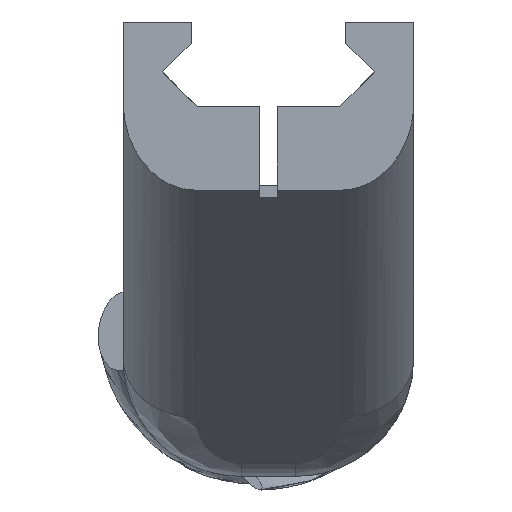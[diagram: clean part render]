
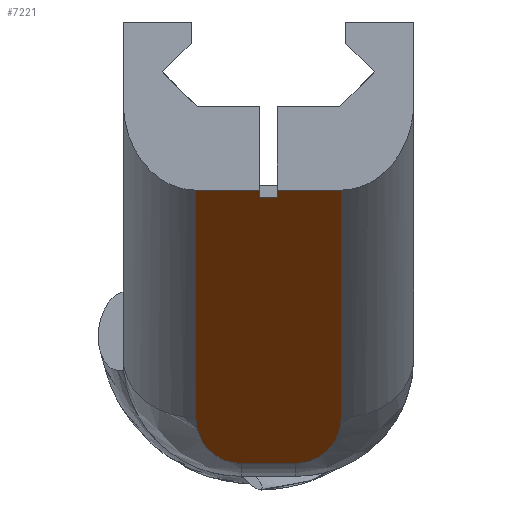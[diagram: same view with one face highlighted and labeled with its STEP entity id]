
A CAD part, front view. The second image highlights one B-rep face of the part: STEP entity #7221.
In plain terms, the highlighted planar face has unit normal (0, -0.574, -0.819).
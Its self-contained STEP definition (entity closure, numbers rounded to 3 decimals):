
#200 = EDGE_CURVE ( 'NONE', #5233, #2700, #1106, .T. ) ;
#331 = CARTESIAN_POINT ( 'NONE',  ( 8., 39.963, -21.482 ) ) ;
#423 = CARTESIAN_POINT ( 'NONE',  ( -1., 1.18, 5.674 ) ) ;
#667 = VERTEX_POINT ( 'NONE', #8123 ) ;
#801 = CARTESIAN_POINT ( 'NONE',  ( 16., 1.18, 5.674 ) ) ;
#875 = CARTESIAN_POINT ( 'NONE',  ( 16., 0., 6.5 ) ) ;
#878 = VECTOR ( 'NONE', #1994, 1000. ) ;
#936 = LINE ( 'NONE', #875, #3476 ) ;
#1106 =( BOUNDED_CURVE ( )  B_SPLINE_CURVE ( 3, ( #1747, #4304, #6349, #9947 ),
 .UNSPECIFIED., .F., .T. ) 
 B_SPLINE_CURVE_WITH_KNOTS ( ( 4, 4 ),
 ( 1.571, 3.142 ),
 .UNSPECIFIED. ) 
 CURVE ( )  GEOMETRIC_REPRESENTATION_ITEM ( )  RATIONAL_B_SPLINE_CURVE ( ( 1., 0.805, 0.805, 1. ) ) 
 REPRESENTATION_ITEM ( '' )  );
#1144 = CARTESIAN_POINT ( 'NONE',  ( 5.929, 42.92, -23.553 ) ) ;
#1277 = AXIS2_PLACEMENT_3D ( 'NONE', #10668, #2596, #5287 ) ;
#1302 = CARTESIAN_POINT ( 'NONE',  ( 3., 42.92, -23.553 ) ) ;
#1432 = VERTEX_POINT ( 'NONE', #423 ) ;
#1663 = ORIENTED_EDGE ( 'NONE', *, *, #2831, .T. ) ;
#1701 = DIRECTION ( 'NONE',  ( -1., 0., 0. ) ) ;
#1747 = CARTESIAN_POINT ( 'NONE',  ( -8., 35.78, -18.553 ) ) ;
#1974 = DIRECTION ( 'NONE',  ( 0., -0.819, 0.574 ) ) ;
#1994 = DIRECTION ( 'NONE',  ( 1., 0., 0. ) ) ;
#2178 =( BOUNDED_CURVE ( )  B_SPLINE_CURVE ( 3, ( #6588, #1144, #331, #3803 ),
 .UNSPECIFIED., .F., .T. ) 
 B_SPLINE_CURVE_WITH_KNOTS ( ( 4, 4 ),
 ( 0., 1.571 ),
 .UNSPECIFIED. ) 
 CURVE ( )  GEOMETRIC_REPRESENTATION_ITEM ( )  RATIONAL_B_SPLINE_CURVE ( ( 1., 0.805, 0.805, 1. ) ) 
 REPRESENTATION_ITEM ( '' )  );
#2285 = CARTESIAN_POINT ( 'NONE',  ( 1., 0., 6.5 ) ) ;
#2437 = CARTESIAN_POINT ( 'NONE',  ( 16., 0., 6.5 ) ) ;
#2596 = DIRECTION ( 'NONE',  ( 0., 0.574, 0.819 ) ) ;
#2638 = EDGE_CURVE ( 'NONE', #667, #7764, #2783, .T. ) ;
#2700 = VERTEX_POINT ( 'NONE', #7152 ) ;
#2783 = LINE ( 'NONE', #5602, #3852 ) ;
#2831 = EDGE_CURVE ( 'NONE', #9083, #7705, #2854, .T. ) ;
#2854 = LINE ( 'NONE', #7446, #9708 ) ;
#3458 = VERTEX_POINT ( 'NONE', #11297 ) ;
#3476 = VECTOR ( 'NONE', #1701, 1000. ) ;
#3803 = CARTESIAN_POINT ( 'NONE',  ( 8., 35.78, -18.553 ) ) ;
#3852 = VECTOR ( 'NONE', #1974, 1000. ) ;
#4027 = VECTOR ( 'NONE', #5183, 1000. ) ;
#4177 = DIRECTION ( 'NONE',  ( 1., 0., 0. ) ) ;
#4202 = EDGE_CURVE ( 'NONE', #2700, #7666, #10027, .T. ) ;
#4281 = EDGE_CURVE ( 'NONE', #7764, #9083, #936, .T. ) ;
#4304 = CARTESIAN_POINT ( 'NONE',  ( -8., 39.963, -21.482 ) ) ;
#4727 = DIRECTION ( 'NONE',  ( 0., 0.819, -0.574 ) ) ;
#4997 = EDGE_CURVE ( 'NONE', #1432, #7705, #11282, .T. ) ;
#5050 = ORIENTED_EDGE ( 'NONE', *, *, #2638, .T. ) ;
#5065 = EDGE_CURVE ( 'NONE', #5822, #3458, #9645, .T. ) ;
#5183 = DIRECTION ( 'NONE',  ( -1., 0., 0. ) ) ;
#5233 = VERTEX_POINT ( 'NONE', #8159 ) ;
#5287 = DIRECTION ( 'NONE',  ( 0., -0.819, 0.574 ) ) ;
#5555 = VECTOR ( 'NONE', #7245, 1000. ) ;
#5602 = CARTESIAN_POINT ( 'NONE',  ( 8., 50., -28.51 ) ) ;
#5822 = VERTEX_POINT ( 'NONE', #10461 ) ;
#6167 = FACE_OUTER_BOUND ( 'NONE', #9370, .T. ) ;
#6207 = CARTESIAN_POINT ( 'NONE',  ( 8., 0., 6.5 ) ) ;
#6349 = CARTESIAN_POINT ( 'NONE',  ( -5.929, 42.92, -23.553 ) ) ;
#6436 = LINE ( 'NONE', #8928, #6712 ) ;
#6588 = CARTESIAN_POINT ( 'NONE',  ( 3., 42.92, -23.553 ) ) ;
#6712 = VECTOR ( 'NONE', #11313, 1000. ) ;
#6910 = ORIENTED_EDGE ( 'NONE', *, *, #5065, .T. ) ;
#6945 = ORIENTED_EDGE ( 'NONE', *, *, #4281, .T. ) ;
#7152 = CARTESIAN_POINT ( 'NONE',  ( -3., 42.92, -23.553 ) ) ;
#7221 = ADVANCED_FACE ( 'NONE', ( #6167 ), #10605, .F. ) ;
#7245 = DIRECTION ( 'NONE',  ( 0., 0.819, -0.574 ) ) ;
#7446 = CARTESIAN_POINT ( 'NONE',  ( 1., 50., -28.51 ) ) ;
#7520 = EDGE_CURVE ( 'NONE', #3458, #5233, #11586, .T. ) ;
#7627 = VECTOR ( 'NONE', #4177, 1000. ) ;
#7666 = VERTEX_POINT ( 'NONE', #9731 ) ;
#7705 = VERTEX_POINT ( 'NONE', #10064 ) ;
#7764 = VERTEX_POINT ( 'NONE', #6207 ) ;
#8113 = ORIENTED_EDGE ( 'NONE', *, *, #200, .T. ) ;
#8123 = CARTESIAN_POINT ( 'NONE',  ( 8., 35.78, -18.553 ) ) ;
#8159 = CARTESIAN_POINT ( 'NONE',  ( -8., 35.78, -18.553 ) ) ;
#8339 = ORIENTED_EDGE ( 'NONE', *, *, #4997, .F. ) ;
#8915 = ORIENTED_EDGE ( 'NONE', *, *, #9459, .T. ) ;
#8928 = CARTESIAN_POINT ( 'NONE',  ( -1., 50., -28.51 ) ) ;
#8930 = EDGE_CURVE ( 'NONE', #1432, #5822, #6436, .T. ) ;
#9083 = VERTEX_POINT ( 'NONE', #2285 ) ;
#9370 = EDGE_LOOP ( 'NONE', ( #8339, #11585, #6910, #9466, #8113, #9525, #8915, #5050, #6945, #1663 ) ) ;
#9459 = EDGE_CURVE ( 'NONE', #7666, #667, #2178, .T. ) ;
#9466 = ORIENTED_EDGE ( 'NONE', *, *, #7520, .T. ) ;
#9525 = ORIENTED_EDGE ( 'NONE', *, *, #4202, .T. ) ;
#9645 = LINE ( 'NONE', #2437, #4027 ) ;
#9708 = VECTOR ( 'NONE', #4727, 1000. ) ;
#9731 = CARTESIAN_POINT ( 'NONE',  ( 3., 42.92, -23.553 ) ) ;
#9839 = CARTESIAN_POINT ( 'NONE',  ( -8., 26.421, -12. ) ) ;
#9947 = CARTESIAN_POINT ( 'NONE',  ( -3., 42.92, -23.553 ) ) ;
#10027 = LINE ( 'NONE', #1302, #878 ) ;
#10064 = CARTESIAN_POINT ( 'NONE',  ( 1., 1.18, 5.674 ) ) ;
#10461 = CARTESIAN_POINT ( 'NONE',  ( -1., 0., 6.5 ) ) ;
#10605 = PLANE ( 'NONE',  #1277 ) ;
#10668 = CARTESIAN_POINT ( 'NONE',  ( 16., 50., -28.51 ) ) ;
#11282 = LINE ( 'NONE', #801, #7627 ) ;
#11297 = CARTESIAN_POINT ( 'NONE',  ( -8., 0., 6.5 ) ) ;
#11313 = DIRECTION ( 'NONE',  ( 0., -0.819, 0.574 ) ) ;
#11585 = ORIENTED_EDGE ( 'NONE', *, *, #8930, .T. ) ;
#11586 = LINE ( 'NONE', #9839, #5555 ) ;
